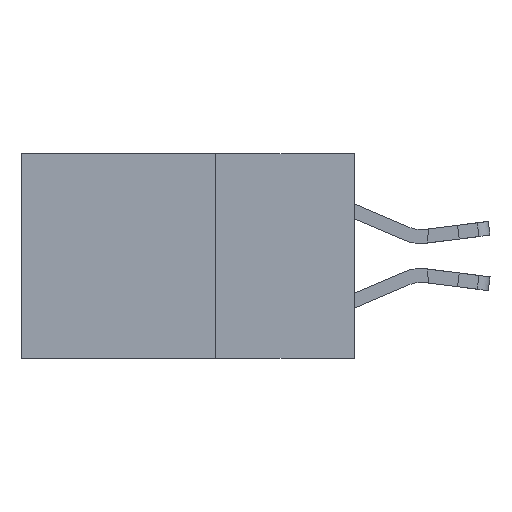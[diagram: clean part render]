
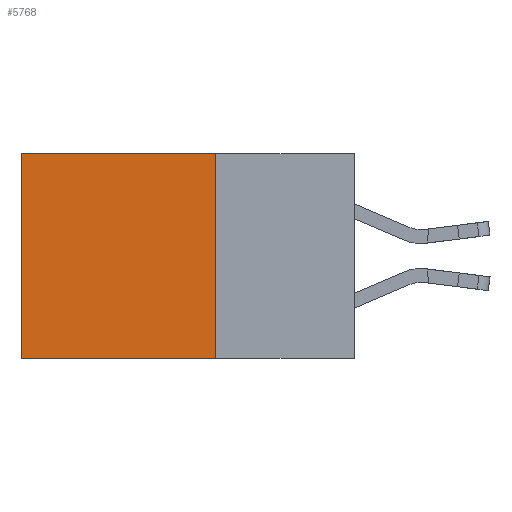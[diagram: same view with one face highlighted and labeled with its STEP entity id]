
A CAD part, left-side view. The second image highlights one B-rep face of the part: STEP entity #5768.
In plain terms, the highlighted planar face has unit normal (-1, 0, 0).
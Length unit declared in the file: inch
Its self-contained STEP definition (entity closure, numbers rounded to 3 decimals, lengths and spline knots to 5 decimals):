
#19 = EDGE_CURVE ( 'NONE', #8225, #4734, #4358, .T. ) ;
#817 = ORIENTED_EDGE ( 'NONE', *, *, #1982, .F. ) ;
#908 = PLANE ( 'NONE',  #7453 ) ;
#1047 = ORIENTED_EDGE ( 'NONE', *, *, #2759, .F. ) ;
#1346 = EDGE_LOOP ( 'NONE', ( #4978, #817, #1047, #7130 ) ) ;
#1913 = VECTOR ( 'NONE', #11222, 39.37008 ) ;
#1925 = CARTESIAN_POINT ( 'NONE',  ( 0.2615, 0.6, -0.37 ) ) ;
#1982 = EDGE_CURVE ( 'NONE', #10598, #9896, #7712, .T. ) ;
#2443 = CARTESIAN_POINT ( 'NONE',  ( 0.2615, 0.6, 0. ) ) ;
#2653 = CARTESIAN_POINT ( 'NONE',  ( 0.2615, 0.25, -0.37 ) ) ;
#2706 = DIRECTION ( 'NONE',  ( 0., 1., 0. ) ) ;
#2759 = EDGE_CURVE ( 'NONE', #8225, #10598, #9511, .T. ) ;
#4019 = VECTOR ( 'NONE', #4936, 39.37008 ) ;
#4198 = DIRECTION ( 'NONE',  ( 0., 0., -1. ) ) ;
#4358 = LINE ( 'NONE', #8305, #11501 ) ;
#4734 = VERTEX_POINT ( 'NONE', #2443 ) ;
#4884 = EDGE_CURVE ( 'NONE', #4734, #9896, #11497, .T. ) ;
#4936 = DIRECTION ( 'NONE',  ( 0., 0., -1. ) ) ;
#4978 = ORIENTED_EDGE ( 'NONE', *, *, #4884, .T. ) ;
#5768 = ADVANCED_FACE ( 'NONE', ( #8280 ), #908, .F. ) ;
#6233 = CARTESIAN_POINT ( 'NONE',  ( 0.2615, 0.25, -0.37 ) ) ;
#7130 = ORIENTED_EDGE ( 'NONE', *, *, #19, .T. ) ;
#7453 = AXIS2_PLACEMENT_3D ( 'NONE', #6233, #9895, #4198 ) ;
#7712 = LINE ( 'NONE', #2653, #10092 ) ;
#8225 = VERTEX_POINT ( 'NONE', #11841 ) ;
#8280 = FACE_OUTER_BOUND ( 'NONE', #1346, .T. ) ;
#8305 = CARTESIAN_POINT ( 'NONE',  ( 0.2615, 0.25, 0. ) ) ;
#9511 = LINE ( 'NONE', #10337, #1913 ) ;
#9895 = DIRECTION ( 'NONE',  ( 1., 0., 0. ) ) ;
#9896 = VERTEX_POINT ( 'NONE', #1925 ) ;
#9974 = DIRECTION ( 'NONE',  ( 0., 1., 0. ) ) ;
#10092 = VECTOR ( 'NONE', #2706, 39.37008 ) ;
#10337 = CARTESIAN_POINT ( 'NONE',  ( 0.2615, 0.25, -0.37 ) ) ;
#10348 = CARTESIAN_POINT ( 'NONE',  ( 0.2615, 0.25, -0.37 ) ) ;
#10598 = VERTEX_POINT ( 'NONE', #10348 ) ;
#11222 = DIRECTION ( 'NONE',  ( 0., 0., -1. ) ) ;
#11392 = CARTESIAN_POINT ( 'NONE',  ( 0.2615, 0.6, -0.37 ) ) ;
#11497 = LINE ( 'NONE', #11392, #4019 ) ;
#11501 = VECTOR ( 'NONE', #9974, 39.37008 ) ;
#11841 = CARTESIAN_POINT ( 'NONE',  ( 0.2615, 0.25, 0. ) ) ;
